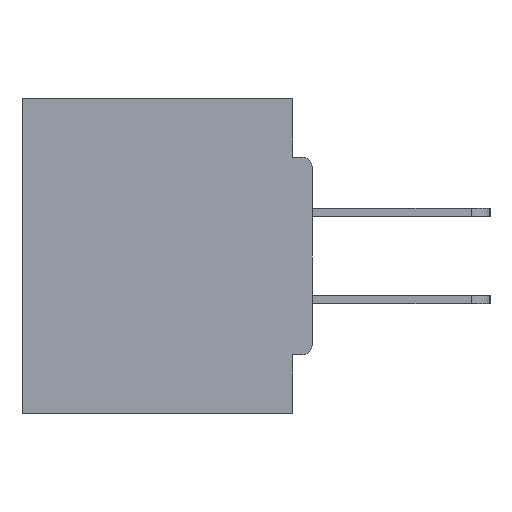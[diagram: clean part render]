
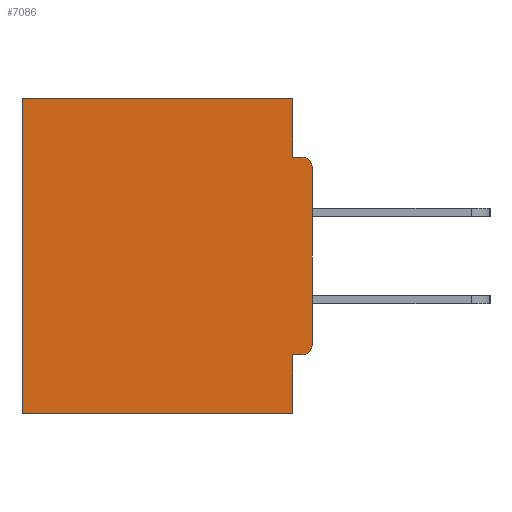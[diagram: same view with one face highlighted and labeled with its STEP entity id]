
A CAD part, left-side view. The second image highlights one B-rep face of the part: STEP entity #7086.
In plain terms, the highlighted planar face has unit normal (-1, 0, 0).
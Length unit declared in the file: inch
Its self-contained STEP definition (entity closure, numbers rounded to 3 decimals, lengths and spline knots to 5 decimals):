
#764 = DIRECTION ( 'NONE',  ( 0., 0., -1. ) ) ;
#1871 = CARTESIAN_POINT ( 'NONE',  ( 0.298, 0.015, -0.3915 ) ) ;
#2172 = VECTOR ( 'NONE', #16024, 39.37008 ) ;
#2254 = VECTOR ( 'NONE', #31629, 39.37008 ) ;
#2698 = VERTEX_POINT ( 'NONE', #23722 ) ;
#3274 = VECTOR ( 'NONE', #25716, 39.37008 ) ;
#3520 = PLANE ( 'NONE',  #32470 ) ;
#3761 = ORIENTED_EDGE ( 'NONE', *, *, #13016, .T. ) ;
#4084 = DIRECTION ( 'NONE',  ( 0., 1., 0. ) ) ;
#4362 = CARTESIAN_POINT ( 'NONE',  ( 0.298, 0., 0. ) ) ;
#5104 = EDGE_CURVE ( 'NONE', #11437, #25900, #5413, .T. ) ;
#5147 = ORIENTED_EDGE ( 'NONE', *, *, #19887, .F. ) ;
#5223 = DIRECTION ( 'NONE',  ( -1., 0., 0. ) ) ;
#5322 = VERTEX_POINT ( 'NONE', #30155 ) ;
#5385 = ORIENTED_EDGE ( 'NONE', *, *, #32213, .T. ) ;
#5413 = LINE ( 'NONE', #6419, #22042 ) ;
#5510 = LINE ( 'NONE', #11301, #25253 ) ;
#5598 = VECTOR ( 'NONE', #27006, 39.37008 ) ;
#6249 = EDGE_CURVE ( 'NONE', #28887, #14159, #6537, .T. ) ;
#6419 = CARTESIAN_POINT ( 'NONE',  ( 0.298, 0., 0. ) ) ;
#6468 = FACE_OUTER_BOUND ( 'NONE', #11565, .T. ) ;
#6537 = LINE ( 'NONE', #16129, #2172 ) ;
#6585 = CARTESIAN_POINT ( 'NONE',  ( 0.298, 0.031, -0.4065 ) ) ;
#6989 = EDGE_CURVE ( 'NONE', #11437, #22599, #18663, .T. ) ;
#7086 = ADVANCED_FACE ( 'NONE', ( #6468 ), #3520, .F. ) ;
#7875 = CARTESIAN_POINT ( 'NONE',  ( 0.298, 0.015, -0.1085 ) ) ;
#8015 = ORIENTED_EDGE ( 'NONE', *, *, #5104, .T. ) ;
#8065 = CARTESIAN_POINT ( 'NONE',  ( 0.298, 0.031, -0.5 ) ) ;
#10863 = ORIENTED_EDGE ( 'NONE', *, *, #19648, .F. ) ;
#11301 = CARTESIAN_POINT ( 'NONE',  ( 0.298, 0.46, 0. ) ) ;
#11437 = VERTEX_POINT ( 'NONE', #29531 ) ;
#11565 = EDGE_LOOP ( 'NONE', ( #5385, #29945, #12420, #8015, #3761, #5147, #12293, #23083, #27008, #10863 ) ) ;
#12293 = ORIENTED_EDGE ( 'NONE', *, *, #6249, .F. ) ;
#12420 = ORIENTED_EDGE ( 'NONE', *, *, #6989, .F. ) ;
#12718 = DIRECTION ( 'NONE',  ( 0., 0., -1. ) ) ;
#13016 = EDGE_CURVE ( 'NONE', #25900, #29801, #5510, .T. ) ;
#13499 = CIRCLE ( 'NONE', #26210, 0.015 ) ;
#13864 = DIRECTION ( 'NONE',  ( 0., 0., -1. ) ) ;
#14159 = VERTEX_POINT ( 'NONE', #24410 ) ;
#14940 = CARTESIAN_POINT ( 'NONE',  ( 0.298, 0., -0.5 ) ) ;
#14963 = EDGE_CURVE ( 'NONE', #22599, #21687, #15675, .T. ) ;
#15675 = LINE ( 'NONE', #24003, #2254 ) ;
#16024 = DIRECTION ( 'NONE',  ( 0., 0., -1. ) ) ;
#16129 = CARTESIAN_POINT ( 'NONE',  ( 0.298, 0.031, -0.5 ) ) ;
#16894 = CARTESIAN_POINT ( 'NONE',  ( 0.298, 0., -0.4065 ) ) ;
#18663 = LINE ( 'NONE', #8065, #3274 ) ;
#19541 = CARTESIAN_POINT ( 'NONE',  ( 0.298, 0.46, -0.5 ) ) ;
#19648 = EDGE_CURVE ( 'NONE', #5322, #28015, #26117, .T. ) ;
#19887 = EDGE_CURVE ( 'NONE', #14159, #29801, #20981, .T. ) ;
#20509 = CARTESIAN_POINT ( 'NONE',  ( 0.298, 0.015, -0.0935 ) ) ;
#20981 = LINE ( 'NONE', #14940, #31634 ) ;
#21687 = VERTEX_POINT ( 'NONE', #20509 ) ;
#22042 = VECTOR ( 'NONE', #28918, 39.37008 ) ;
#22568 = DIRECTION ( 'NONE',  ( 0., 1., 0. ) ) ;
#22599 = VERTEX_POINT ( 'NONE', #29249 ) ;
#23083 = ORIENTED_EDGE ( 'NONE', *, *, #30217, .F. ) ;
#23412 = DIRECTION ( 'NONE',  ( 1., 0., 0. ) ) ;
#23493 = CIRCLE ( 'NONE', #26108, 0.015 ) ;
#23722 = CARTESIAN_POINT ( 'NONE',  ( 0.298, 0.015, -0.4065 ) ) ;
#24003 = CARTESIAN_POINT ( 'NONE',  ( 0.298, 0., -0.0935 ) ) ;
#24410 = CARTESIAN_POINT ( 'NONE',  ( 0.298, 0.031, -0.5 ) ) ;
#25253 = VECTOR ( 'NONE', #13864, 39.37008 ) ;
#25577 = EDGE_CURVE ( 'NONE', #2698, #28015, #13499, .T. ) ;
#25716 = DIRECTION ( 'NONE',  ( 0., 0., -1. ) ) ;
#25900 = VERTEX_POINT ( 'NONE', #32699 ) ;
#26108 = AXIS2_PLACEMENT_3D ( 'NONE', #7875, #5223, #12718 ) ;
#26117 = LINE ( 'NONE', #4362, #5598 ) ;
#26210 = AXIS2_PLACEMENT_3D ( 'NONE', #1871, #27133, #29694 ) ;
#27006 = DIRECTION ( 'NONE',  ( 0., 0., -1. ) ) ;
#27008 = ORIENTED_EDGE ( 'NONE', *, *, #25577, .T. ) ;
#27133 = DIRECTION ( 'NONE',  ( -1., 0., 0. ) ) ;
#28015 = VERTEX_POINT ( 'NONE', #29704 ) ;
#28799 = CARTESIAN_POINT ( 'NONE',  ( 0.298, 0., 0. ) ) ;
#28887 = VERTEX_POINT ( 'NONE', #6585 ) ;
#28918 = DIRECTION ( 'NONE',  ( 0., 1., 0. ) ) ;
#29249 = CARTESIAN_POINT ( 'NONE',  ( 0.298, 0.031, -0.0935 ) ) ;
#29531 = CARTESIAN_POINT ( 'NONE',  ( 0.298, 0.031, 0. ) ) ;
#29694 = DIRECTION ( 'NONE',  ( 0., 0., -1. ) ) ;
#29704 = CARTESIAN_POINT ( 'NONE',  ( 0.298, 0., -0.3915 ) ) ;
#29801 = VERTEX_POINT ( 'NONE', #19541 ) ;
#29945 = ORIENTED_EDGE ( 'NONE', *, *, #14963, .F. ) ;
#30155 = CARTESIAN_POINT ( 'NONE',  ( 0.298, 0., -0.1085 ) ) ;
#30217 = EDGE_CURVE ( 'NONE', #2698, #28887, #31536, .T. ) ;
#30379 = VECTOR ( 'NONE', #4084, 39.37008 ) ;
#31536 = LINE ( 'NONE', #16894, #30379 ) ;
#31629 = DIRECTION ( 'NONE',  ( 0., -1., 0. ) ) ;
#31634 = VECTOR ( 'NONE', #22568, 39.37008 ) ;
#32213 = EDGE_CURVE ( 'NONE', #5322, #21687, #23493, .T. ) ;
#32470 = AXIS2_PLACEMENT_3D ( 'NONE', #28799, #23412, #764 ) ;
#32699 = CARTESIAN_POINT ( 'NONE',  ( 0.298, 0.46, 0. ) ) ;
